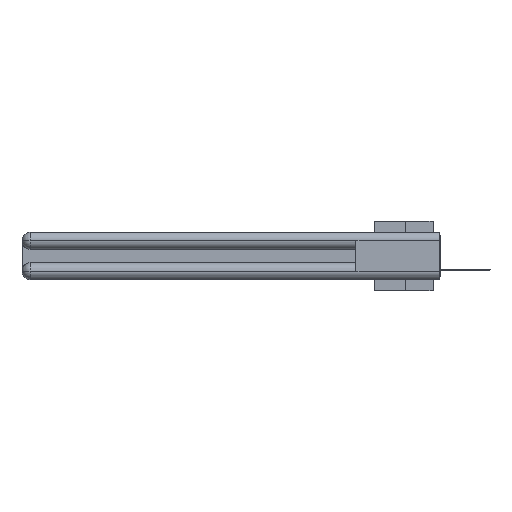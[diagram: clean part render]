
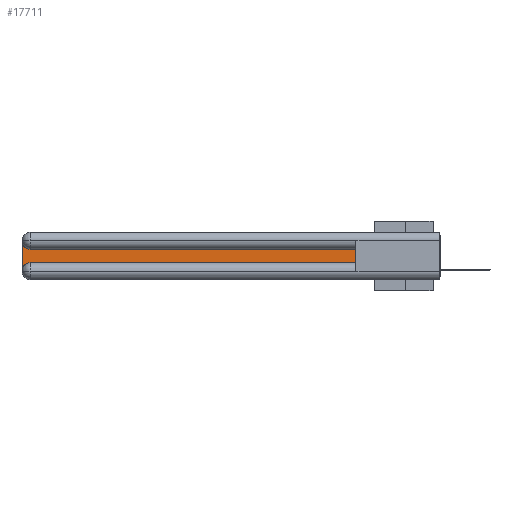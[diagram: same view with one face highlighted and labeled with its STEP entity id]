
A CAD part, left-side view. The second image highlights one B-rep face of the part: STEP entity #17711.
In plain terms, the highlighted planar face has unit normal (-1, 0, 0).
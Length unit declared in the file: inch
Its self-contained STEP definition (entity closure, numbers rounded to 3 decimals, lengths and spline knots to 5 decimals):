
#392 = VECTOR ( 'NONE', #4857, 39.37008 ) ;
#894 = VERTEX_POINT ( 'NONE', #19379 ) ;
#1159 = CARTESIAN_POINT ( 'NONE',  ( 0.075, 3., -0.1225 ) ) ;
#1242 = CIRCLE ( 'NONE', #18906, 0.06 ) ;
#1955 = EDGE_CURVE ( 'NONE', #14732, #6645, #21454, .T. ) ;
#2000 = CARTESIAN_POINT ( 'NONE',  ( 0.075, 0.6, -0.1225 ) ) ;
#2027 = DIRECTION ( 'NONE',  ( 1., 0., 0. ) ) ;
#2492 = DIRECTION ( 'NONE',  ( 0., 0., -1. ) ) ;
#2592 = VECTOR ( 'NONE', #13476, 39.37008 ) ;
#2642 = EDGE_LOOP ( 'NONE', ( #17100, #27065, #8758, #3483, #9047, #17582 ) ) ;
#2926 = VERTEX_POINT ( 'NONE', #8370 ) ;
#3140 = VECTOR ( 'NONE', #13796, 39.37008 ) ;
#3476 = EDGE_CURVE ( 'NONE', #23832, #14732, #25654, .T. ) ;
#3483 = ORIENTED_EDGE ( 'NONE', *, *, #23266, .T. ) ;
#3917 = AXIS2_PLACEMENT_3D ( 'NONE', #16151, #25804, #4140 ) ;
#4140 = DIRECTION ( 'NONE',  ( 0., 0., -1. ) ) ;
#4492 = EDGE_CURVE ( 'NONE', #17136, #894, #23299, .T. ) ;
#4627 = VECTOR ( 'NONE', #30963, 39.37008 ) ;
#4857 = DIRECTION ( 'NONE',  ( 0., 1., 0. ) ) ;
#6450 = CARTESIAN_POINT ( 'NONE',  ( 0.075, 0.6, -0.2175 ) ) ;
#6645 = VERTEX_POINT ( 'NONE', #20476 ) ;
#8370 = CARTESIAN_POINT ( 'NONE',  ( 0.075, 2.94, -0.2175 ) ) ;
#8738 = PLANE ( 'NONE',  #29826 ) ;
#8758 = ORIENTED_EDGE ( 'NONE', *, *, #4492, .T. ) ;
#9047 = ORIENTED_EDGE ( 'NONE', *, *, #18646, .T. ) ;
#11977 = CARTESIAN_POINT ( 'NONE',  ( 0.075, 2.94, -0.2775 ) ) ;
#13008 = DIRECTION ( 'NONE',  ( 1., 0., 0. ) ) ;
#13476 = DIRECTION ( 'NONE',  ( 0., 0., 1. ) ) ;
#13550 = LINE ( 'NONE', #6450, #4627 ) ;
#13796 = DIRECTION ( 'NONE',  ( 0., 0., -1. ) ) ;
#14732 = VERTEX_POINT ( 'NONE', #26693 ) ;
#15021 = CIRCLE ( 'NONE', #3917, 0.06 ) ;
#16151 = CARTESIAN_POINT ( 'NONE',  ( 0.075, 2.94, -0.0625 ) ) ;
#17100 = ORIENTED_EDGE ( 'NONE', *, *, #1955, .T. ) ;
#17136 = VERTEX_POINT ( 'NONE', #27994 ) ;
#17582 = ORIENTED_EDGE ( 'NONE', *, *, #3476, .T. ) ;
#17711 = ADVANCED_FACE ( 'NONE', ( #17750 ), #8738, .F. ) ;
#17750 = FACE_OUTER_BOUND ( 'NONE', #2642, .T. ) ;
#18646 = EDGE_CURVE ( 'NONE', #2926, #23832, #13550, .T. ) ;
#18906 = AXIS2_PLACEMENT_3D ( 'NONE', #11977, #2027, #2492 ) ;
#19379 = CARTESIAN_POINT ( 'NONE',  ( 0.075, 3., -0.2775 ) ) ;
#20476 = CARTESIAN_POINT ( 'NONE',  ( 0.075, 2.94, -0.1225 ) ) ;
#21454 = LINE ( 'NONE', #2000, #392 ) ;
#23266 = EDGE_CURVE ( 'NONE', #894, #2926, #1242, .T. ) ;
#23299 = LINE ( 'NONE', #25658, #3140 ) ;
#23832 = VERTEX_POINT ( 'NONE', #30790 ) ;
#25654 = LINE ( 'NONE', #28198, #2592 ) ;
#25658 = CARTESIAN_POINT ( 'NONE',  ( 0.075, 3., -0.2175 ) ) ;
#25804 = DIRECTION ( 'NONE',  ( 1., 0., 0. ) ) ;
#26017 = EDGE_CURVE ( 'NONE', #6645, #17136, #15021, .T. ) ;
#26693 = CARTESIAN_POINT ( 'NONE',  ( 0.075, 0.6, -0.1225 ) ) ;
#27065 = ORIENTED_EDGE ( 'NONE', *, *, #26017, .T. ) ;
#27562 = DIRECTION ( 'NONE',  ( 0., 0., -1. ) ) ;
#27994 = CARTESIAN_POINT ( 'NONE',  ( 0.075, 3., -0.0625 ) ) ;
#28198 = CARTESIAN_POINT ( 'NONE',  ( 0.075, 0.6, -0.2175 ) ) ;
#29826 = AXIS2_PLACEMENT_3D ( 'NONE', #1159, #13008, #27562 ) ;
#30790 = CARTESIAN_POINT ( 'NONE',  ( 0.075, 0.6, -0.2175 ) ) ;
#30963 = DIRECTION ( 'NONE',  ( 0., -1., 0. ) ) ;
